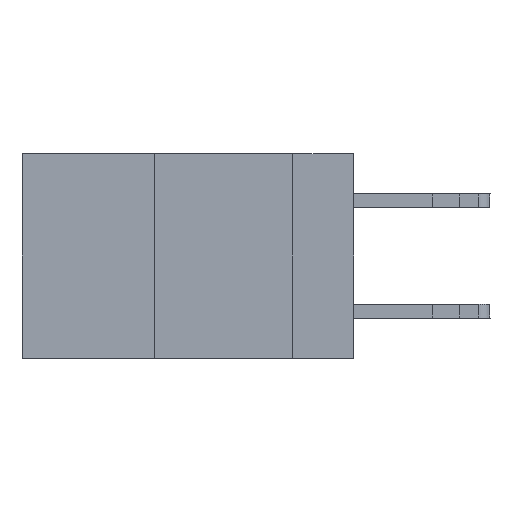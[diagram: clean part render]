
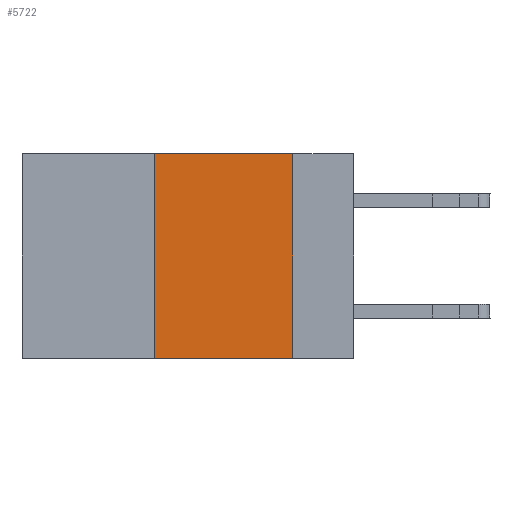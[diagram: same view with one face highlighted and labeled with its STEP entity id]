
A CAD part, left-side view. The second image highlights one B-rep face of the part: STEP entity #5722.
In plain terms, the highlighted planar face has unit normal (-1, 0, 0).
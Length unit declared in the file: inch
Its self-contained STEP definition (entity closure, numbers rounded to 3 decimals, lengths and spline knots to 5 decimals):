
#462 = LINE ( 'NONE', #20058, #2857 ) ;
#941 = CARTESIAN_POINT ( 'NONE',  ( 0., 0.6, 0. ) ) ;
#1221 = CARTESIAN_POINT ( 'NONE',  ( 0., 0.11, 0. ) ) ;
#2507 = DIRECTION ( 'NONE',  ( 0., 0., -1. ) ) ;
#2857 = VECTOR ( 'NONE', #2507, 39.37008 ) ;
#3220 = CARTESIAN_POINT ( 'NONE',  ( 0., 0.36, 0. ) ) ;
#4232 = EDGE_CURVE ( 'NONE', #16401, #13523, #8044, .T. ) ;
#4259 = VECTOR ( 'NONE', #10616, 39.37008 ) ;
#4368 = EDGE_CURVE ( 'NONE', #10702, #16401, #5209, .T. ) ;
#4626 = VECTOR ( 'NONE', #22070, 39.37008 ) ;
#5209 = LINE ( 'NONE', #3220, #4259 ) ;
#5722 = ADVANCED_FACE ( 'NONE', ( #8847 ), #14804, .F. ) ;
#5889 = ORIENTED_EDGE ( 'NONE', *, *, #4368, .F. ) ;
#6680 = VERTEX_POINT ( 'NONE', #14140 ) ;
#6966 = VECTOR ( 'NONE', #16464, 39.37008 ) ;
#7563 = CARTESIAN_POINT ( 'NONE',  ( 0., 0.6, 0. ) ) ;
#8044 = LINE ( 'NONE', #941, #4626 ) ;
#8620 = EDGE_LOOP ( 'NONE', ( #14778, #16400, #5889, #12715 ) ) ;
#8847 = FACE_OUTER_BOUND ( 'NONE', #8620, .T. ) ;
#8848 = CARTESIAN_POINT ( 'NONE',  ( 0., 0.36, 0. ) ) ;
#10616 = DIRECTION ( 'NONE',  ( 0., 0., 1. ) ) ;
#10702 = VERTEX_POINT ( 'NONE', #17914 ) ;
#11210 = CARTESIAN_POINT ( 'NONE',  ( 0., 0.6, -0.37 ) ) ;
#11313 = DIRECTION ( 'NONE',  ( 0., 0., -1. ) ) ;
#11556 = LINE ( 'NONE', #11210, #6966 ) ;
#12715 = ORIENTED_EDGE ( 'NONE', *, *, #21021, .T. ) ;
#13523 = VERTEX_POINT ( 'NONE', #1221 ) ;
#14140 = CARTESIAN_POINT ( 'NONE',  ( 0., 0.11, -0.37 ) ) ;
#14778 = ORIENTED_EDGE ( 'NONE', *, *, #22896, .F. ) ;
#14804 = PLANE ( 'NONE',  #22614 ) ;
#16343 = DIRECTION ( 'NONE',  ( 1., 0., 0. ) ) ;
#16400 = ORIENTED_EDGE ( 'NONE', *, *, #4232, .F. ) ;
#16401 = VERTEX_POINT ( 'NONE', #8848 ) ;
#16464 = DIRECTION ( 'NONE',  ( 0., -1., 0. ) ) ;
#17914 = CARTESIAN_POINT ( 'NONE',  ( 0., 0.36, -0.37 ) ) ;
#20058 = CARTESIAN_POINT ( 'NONE',  ( 0., 0.11, 0. ) ) ;
#21021 = EDGE_CURVE ( 'NONE', #10702, #6680, #11556, .T. ) ;
#22070 = DIRECTION ( 'NONE',  ( 0., -1., 0. ) ) ;
#22614 = AXIS2_PLACEMENT_3D ( 'NONE', #7563, #16343, #11313 ) ;
#22896 = EDGE_CURVE ( 'NONE', #13523, #6680, #462, .T. ) ;
